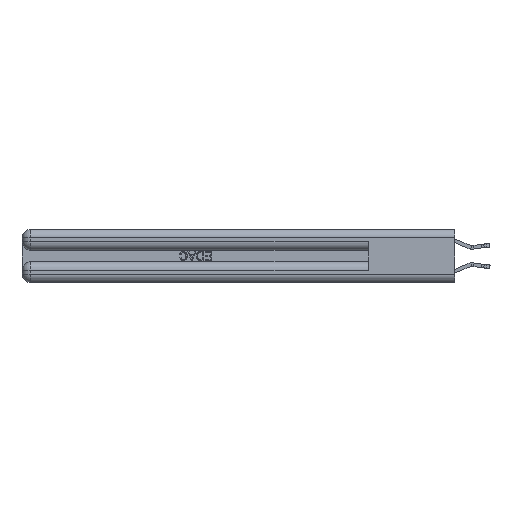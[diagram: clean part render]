
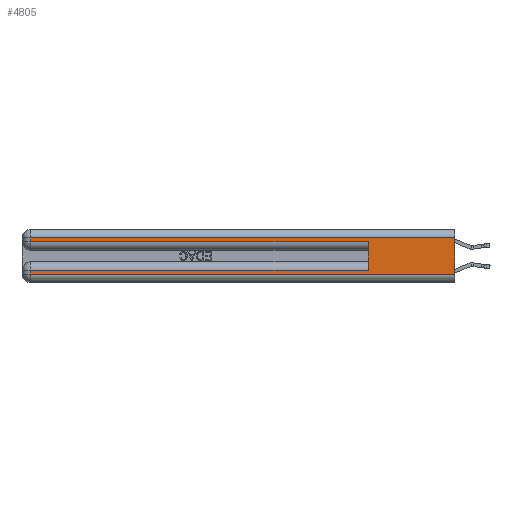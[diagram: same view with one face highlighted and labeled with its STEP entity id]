
A CAD part, left-side view. The second image highlights one B-rep face of the part: STEP entity #4805.
In plain terms, the highlighted planar face has unit normal (-1, 0, 0).
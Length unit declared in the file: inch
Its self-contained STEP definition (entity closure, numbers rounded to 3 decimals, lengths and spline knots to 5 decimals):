
#4 = VECTOR ( 'NONE', #31336, 39.37008 ) ;
#111 = LINE ( 'NONE', #27457, #25625 ) ;
#113 = VECTOR ( 'NONE', #19483, 39.37008 ) ;
#1021 = EDGE_CURVE ( 'NONE', #21034, #15712, #111, .T. ) ;
#1701 = CARTESIAN_POINT ( 'NONE',  ( 0., 0.6, 0.285 ) ) ;
#1859 = VECTOR ( 'NONE', #25808, 39.37008 ) ;
#2137 = CARTESIAN_POINT ( 'NONE',  ( 0., 2.94, 0.085 ) ) ;
#2388 = EDGE_CURVE ( 'NONE', #19029, #30212, #17262, .T. ) ;
#2881 = DIRECTION ( 'NONE',  ( 0., 0., -1. ) ) ;
#3120 = AXIS2_PLACEMENT_3D ( 'NONE', #21933, #19488, #13266 ) ;
#3393 = ORIENTED_EDGE ( 'NONE', *, *, #15962, .F. ) ;
#4443 = ORIENTED_EDGE ( 'NONE', *, *, #26345, .T. ) ;
#4779 = ORIENTED_EDGE ( 'NONE', *, *, #2388, .F. ) ;
#4805 = ADVANCED_FACE ( 'NONE', ( #11397 ), #24726, .F. ) ;
#5959 = VERTEX_POINT ( 'NONE', #34242 ) ;
#6406 = LINE ( 'NONE', #14364, #1859 ) ;
#6634 = EDGE_CURVE ( 'NONE', #13733, #26614, #22176, .T. ) ;
#7446 = DIRECTION ( 'NONE',  ( 0., 0., -1. ) ) ;
#9038 = VECTOR ( 'NONE', #31820, 39.37008 ) ;
#9292 = DIRECTION ( 'NONE',  ( 0., 0., -1. ) ) ;
#9328 = ORIENTED_EDGE ( 'NONE', *, *, #26143, .T. ) ;
#11397 = FACE_OUTER_BOUND ( 'NONE', #17106, .T. ) ;
#11498 = CARTESIAN_POINT ( 'NONE',  ( 0., 0.6, 0.145 ) ) ;
#13266 = DIRECTION ( 'NONE',  ( 0., 0., -1. ) ) ;
#13455 = CARTESIAN_POINT ( 'NONE',  ( 0., 0., 0.31 ) ) ;
#13733 = VERTEX_POINT ( 'NONE', #21352 ) ;
#14041 = LINE ( 'NONE', #11498, #18690 ) ;
#14364 = CARTESIAN_POINT ( 'NONE',  ( 0., 0., 0.085 ) ) ;
#14739 = ORIENTED_EDGE ( 'NONE', *, *, #32933, .T. ) ;
#15712 = VERTEX_POINT ( 'NONE', #28579 ) ;
#15962 = EDGE_CURVE ( 'NONE', #21936, #26614, #14041, .T. ) ;
#16286 = ORIENTED_EDGE ( 'NONE', *, *, #6634, .T. ) ;
#17106 = EDGE_LOOP ( 'NONE', ( #4779, #23537, #14739, #16286, #3393, #9328, #25460, #4443 ) ) ;
#17262 = LINE ( 'NONE', #28398, #30527 ) ;
#18130 = CARTESIAN_POINT ( 'NONE',  ( 0., 0., 0.06 ) ) ;
#18690 = VECTOR ( 'NONE', #29889, 39.37008 ) ;
#19029 = VERTEX_POINT ( 'NONE', #13455 ) ;
#19483 = DIRECTION ( 'NONE',  ( 0., -1., 0. ) ) ;
#19488 = DIRECTION ( 'NONE',  ( 1., 0., 0. ) ) ;
#21034 = VERTEX_POINT ( 'NONE', #2137 ) ;
#21352 = CARTESIAN_POINT ( 'NONE',  ( 0., 2.94, 0.285 ) ) ;
#21726 = LINE ( 'NONE', #23458, #30818 ) ;
#21933 = CARTESIAN_POINT ( 'NONE',  ( 0., 0., 0.37 ) ) ;
#21936 = VERTEX_POINT ( 'NONE', #24933 ) ;
#22032 = LINE ( 'NONE', #28956, #9038 ) ;
#22176 = LINE ( 'NONE', #25681, #4 ) ;
#23458 = CARTESIAN_POINT ( 'NONE',  ( 0., 2.94, 0.37 ) ) ;
#23537 = ORIENTED_EDGE ( 'NONE', *, *, #31015, .T. ) ;
#24726 = PLANE ( 'NONE',  #3120 ) ;
#24933 = CARTESIAN_POINT ( 'NONE',  ( 0., 0.6, 0.085 ) ) ;
#25460 = ORIENTED_EDGE ( 'NONE', *, *, #1021, .T. ) ;
#25625 = VECTOR ( 'NONE', #9292, 39.37008 ) ;
#25681 = CARTESIAN_POINT ( 'NONE',  ( 0., 0., 0.285 ) ) ;
#25808 = DIRECTION ( 'NONE',  ( 0., 1., 0. ) ) ;
#26143 = EDGE_CURVE ( 'NONE', #21936, #21034, #6406, .T. ) ;
#26345 = EDGE_CURVE ( 'NONE', #15712, #30212, #31809, .T. ) ;
#26614 = VERTEX_POINT ( 'NONE', #1701 ) ;
#27442 = CARTESIAN_POINT ( 'NONE',  ( 0., 0., 0.06 ) ) ;
#27457 = CARTESIAN_POINT ( 'NONE',  ( 0., 2.94, 0.37 ) ) ;
#28398 = CARTESIAN_POINT ( 'NONE',  ( 0., 0., 0.37 ) ) ;
#28579 = CARTESIAN_POINT ( 'NONE',  ( 0., 2.94, 0.06 ) ) ;
#28956 = CARTESIAN_POINT ( 'NONE',  ( 0., 0., 0.31 ) ) ;
#29889 = DIRECTION ( 'NONE',  ( 0., 0., 1. ) ) ;
#30212 = VERTEX_POINT ( 'NONE', #18130 ) ;
#30527 = VECTOR ( 'NONE', #2881, 39.37008 ) ;
#30818 = VECTOR ( 'NONE', #7446, 39.37008 ) ;
#31015 = EDGE_CURVE ( 'NONE', #19029, #5959, #22032, .T. ) ;
#31336 = DIRECTION ( 'NONE',  ( 0., -1., 0. ) ) ;
#31809 = LINE ( 'NONE', #27442, #113 ) ;
#31820 = DIRECTION ( 'NONE',  ( 0., 1., 0. ) ) ;
#32933 = EDGE_CURVE ( 'NONE', #5959, #13733, #21726, .T. ) ;
#34242 = CARTESIAN_POINT ( 'NONE',  ( 0., 2.94, 0.31 ) ) ;
